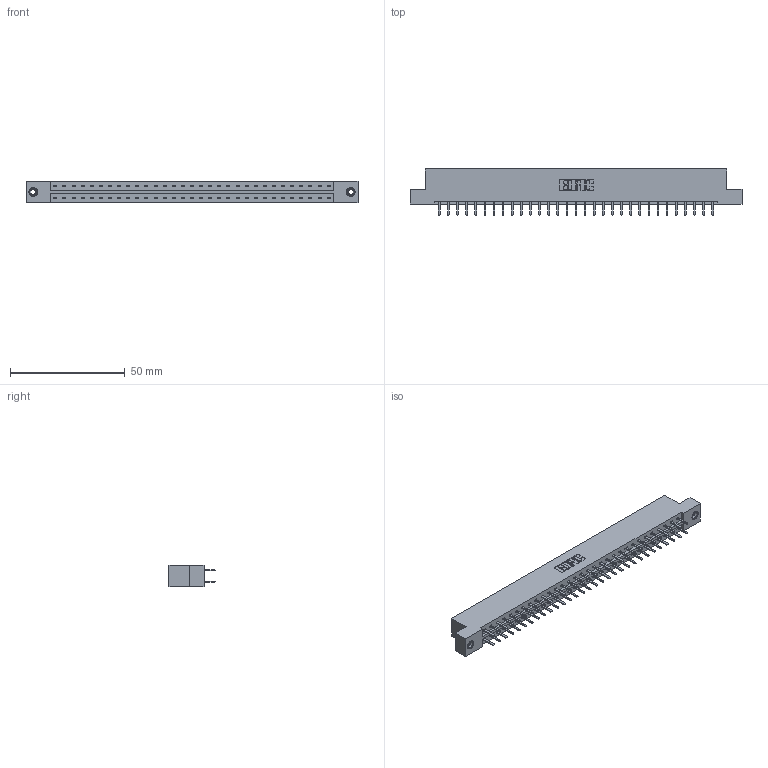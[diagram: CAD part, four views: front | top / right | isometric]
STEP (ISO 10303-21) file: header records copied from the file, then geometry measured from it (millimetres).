
FILE_DESCRIPTION (( 'STEP AP203' ), '1' );
FILE_NAME ('833-062-520-208.STEP', '2020-06-05T05:07:03', ( '' ), ( '' ), 'SwSTEP 2.0', 'SolidWorks 2020', '' );
FILE_SCHEMA (( 'CONFIG_CONTROL_DESIGN' ));
Length unit declared in the file: inch
Products named in the file (4): 833-062-520-208; 345-292-001_345-293-120; 833 Part_Flush - .156 Dia - TI; 345-250-001_345-250-003-102
Assembly tree (65 placements, depth 2):
  833-062-520-208
    833 Part_Flush - .156 Dia - TI
    345-292-001_345-293-120  x62
    345-250-001_345-250-003-102  x2
Bounding box: 144.37 x 20.02 x 9.4 mm (x, y, z)
Volume: 14603.1 mm3; surface area: 17095.8 mm2
Topology: 65 solids, 65 shells, 3646 faces, 10553 edges, 6862 vertices
Faces by surface type: plane 2458, cylinder 1172, cone 12, torus 4
Entity records: 22666 total; most frequent: CARTESIAN_POINT 3765, ORIENTED_EDGE 3682, DIRECTION 3255, EDGE_CURVE 1841, VECTOR 1689, LINE 1689, VERTEX_POINT 1220, AXIS2_PLACEMENT_3D 783
